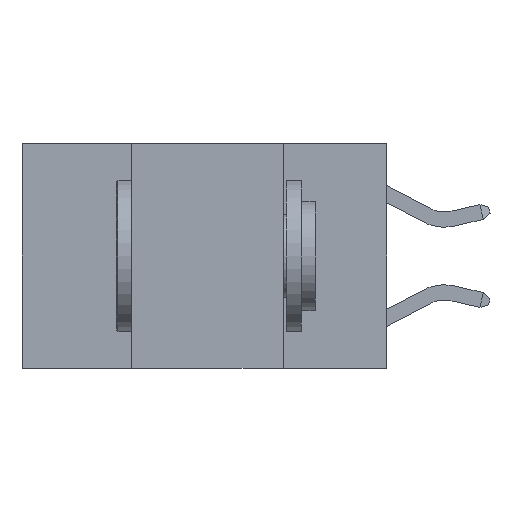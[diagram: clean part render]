
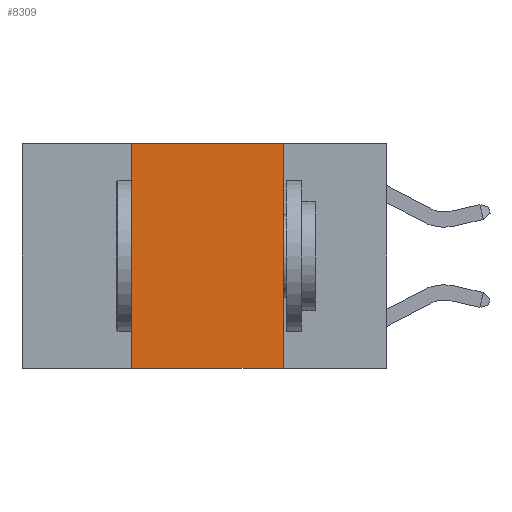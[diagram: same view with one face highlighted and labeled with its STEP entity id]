
A CAD part, left-side view. The second image highlights one B-rep face of the part: STEP entity #8309.
In plain terms, the highlighted planar face has unit normal (-1, 0, 0).
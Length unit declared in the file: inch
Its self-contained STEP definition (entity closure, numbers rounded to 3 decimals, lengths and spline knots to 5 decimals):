
#113 = CARTESIAN_POINT ( 'NONE',  ( 0., 0.17, -0.37 ) ) ;
#327 = VERTEX_POINT ( 'NONE', #6093 ) ;
#375 = VERTEX_POINT ( 'NONE', #113 ) ;
#1066 = VECTOR ( 'NONE', #2577, 39.37008 ) ;
#2251 = VECTOR ( 'NONE', #6273, 39.37008 ) ;
#2577 = DIRECTION ( 'NONE',  ( 0., -1., 0. ) ) ;
#2620 = AXIS2_PLACEMENT_3D ( 'NONE', #10688, #16199, #5247 ) ;
#3195 = CARTESIAN_POINT ( 'NONE',  ( 0., 0.17, 0. ) ) ;
#3381 = VECTOR ( 'NONE', #23132, 39.37008 ) ;
#3435 = PLANE ( 'NONE',  #2620 ) ;
#3919 = LINE ( 'NONE', #3195, #3381 ) ;
#4800 = EDGE_CURVE ( 'NONE', #5808, #375, #10360, .T. ) ;
#5247 = DIRECTION ( 'NONE',  ( 0., 0., -1. ) ) ;
#5401 = VECTOR ( 'NONE', #8928, 39.37008 ) ;
#5808 = VERTEX_POINT ( 'NONE', #11506 ) ;
#6093 = CARTESIAN_POINT ( 'NONE',  ( 0., 0.17, 0. ) ) ;
#6273 = DIRECTION ( 'NONE',  ( 0., -1., 0. ) ) ;
#6542 = EDGE_CURVE ( 'NONE', #13295, #327, #16878, .T. ) ;
#7110 = CARTESIAN_POINT ( 'NONE',  ( 0., 0.42, 0. ) ) ;
#7611 = EDGE_CURVE ( 'NONE', #5808, #13295, #12009, .T. ) ;
#8309 = ADVANCED_FACE ( 'NONE', ( #12259 ), #3435, .F. ) ;
#8500 = ORIENTED_EDGE ( 'NONE', *, *, #7611, .F. ) ;
#8928 = DIRECTION ( 'NONE',  ( 0., 0., 1. ) ) ;
#10360 = LINE ( 'NONE', #13554, #1066 ) ;
#10688 = CARTESIAN_POINT ( 'NONE',  ( 0., 0.6, 0. ) ) ;
#11506 = CARTESIAN_POINT ( 'NONE',  ( 0., 0.42, -0.37 ) ) ;
#11874 = EDGE_LOOP ( 'NONE', ( #12256, #21888, #8500, #18220 ) ) ;
#12009 = LINE ( 'NONE', #7110, #5401 ) ;
#12101 = CARTESIAN_POINT ( 'NONE',  ( 0., 0.42, 0. ) ) ;
#12256 = ORIENTED_EDGE ( 'NONE', *, *, #18602, .F. ) ;
#12259 = FACE_OUTER_BOUND ( 'NONE', #11874, .T. ) ;
#13295 = VERTEX_POINT ( 'NONE', #12101 ) ;
#13554 = CARTESIAN_POINT ( 'NONE',  ( 0., 0.6, -0.37 ) ) ;
#15380 = CARTESIAN_POINT ( 'NONE',  ( 0., 0.6, 0. ) ) ;
#16199 = DIRECTION ( 'NONE',  ( 1., 0., 0. ) ) ;
#16878 = LINE ( 'NONE', #15380, #2251 ) ;
#18220 = ORIENTED_EDGE ( 'NONE', *, *, #4800, .T. ) ;
#18602 = EDGE_CURVE ( 'NONE', #327, #375, #3919, .T. ) ;
#21888 = ORIENTED_EDGE ( 'NONE', *, *, #6542, .F. ) ;
#23132 = DIRECTION ( 'NONE',  ( 0., 0., -1. ) ) ;
